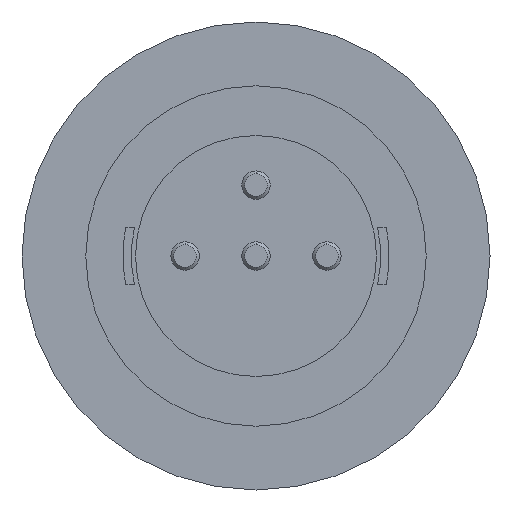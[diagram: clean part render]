
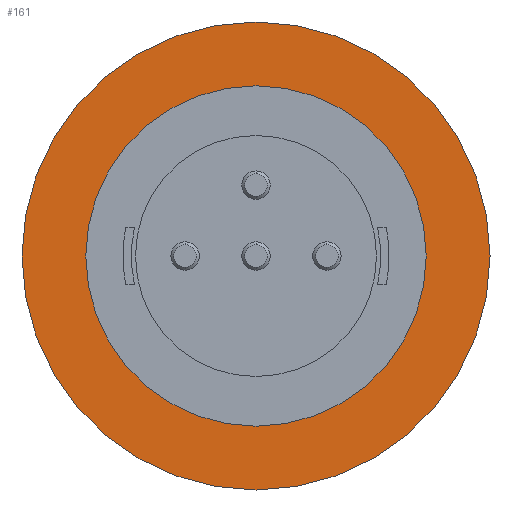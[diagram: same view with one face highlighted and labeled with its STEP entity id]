
A CAD part, front view. The second image highlights one B-rep face of the part: STEP entity #161.
In plain terms, the highlighted planar face has unit normal (0, -1, 0).
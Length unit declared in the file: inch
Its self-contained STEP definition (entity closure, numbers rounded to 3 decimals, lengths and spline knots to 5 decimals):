
#27 = ORIENTED_EDGE ( 'NONE', *, *, #752, .T. ) ;
#47 = AXIS2_PLACEMENT_3D ( 'NONE', #1743, #1665, #1512 ) ;
#58 = CARTESIAN_POINT ( 'NONE',  ( 0., -3.1, 0. ) ) ;
#77 = DIRECTION ( 'NONE',  ( 0., -1., 0. ) ) ;
#83 = AXIS2_PLACEMENT_3D ( 'NONE', #1398, #424, #1243 ) ;
#161 = ADVANCED_FACE ( 'NONE', ( #200, #1588 ), #606, .T. ) ;
#200 = FACE_BOUND ( 'NONE', #368, .T. ) ;
#220 = CARTESIAN_POINT ( 'NONE',  ( 0., -3.1, 8.25 ) ) ;
#285 = CIRCLE ( 'NONE', #1160, 8.25 ) ;
#323 = ORIENTED_EDGE ( 'NONE', *, *, #815, .F. ) ;
#343 = CARTESIAN_POINT ( 'NONE',  ( 0., -3.1, 0. ) ) ;
#368 = EDGE_LOOP ( 'NONE', ( #323, #373 ) ) ;
#373 = ORIENTED_EDGE ( 'NONE', *, *, #448, .F. ) ;
#424 = DIRECTION ( 'NONE',  ( 0., -1., 0. ) ) ;
#448 = EDGE_CURVE ( 'NONE', #1286, #1372, #1666, .T. ) ;
#471 = CARTESIAN_POINT ( 'NONE',  ( 0., -3.1, -8.25 ) ) ;
#606 = PLANE ( 'NONE',  #1515 ) ;
#752 = EDGE_CURVE ( 'NONE', #952, #1498, #285, .T. ) ;
#815 = EDGE_CURVE ( 'NONE', #1372, #1286, #1256, .T. ) ;
#898 = DIRECTION ( 'NONE',  ( 0., 0., -1. ) ) ;
#952 = VERTEX_POINT ( 'NONE', #471 ) ;
#963 = CARTESIAN_POINT ( 'NONE',  ( 0., -3.1, -6. ) ) ;
#1055 = EDGE_LOOP ( 'NONE', ( #1130, #27 ) ) ;
#1130 = ORIENTED_EDGE ( 'NONE', *, *, #1779, .T. ) ;
#1156 = CARTESIAN_POINT ( 'NONE',  ( 0., -3.1, 0. ) ) ;
#1160 = AXIS2_PLACEMENT_3D ( 'NONE', #343, #77, #1209 ) ;
#1193 = DIRECTION ( 'NONE',  ( 0., -1., 0. ) ) ;
#1209 = DIRECTION ( 'NONE',  ( 0., 0., -1. ) ) ;
#1243 = DIRECTION ( 'NONE',  ( 0., 0., -1. ) ) ;
#1256 = CIRCLE ( 'NONE', #47, 6. ) ;
#1283 = AXIS2_PLACEMENT_3D ( 'NONE', #1156, #1193, #1751 ) ;
#1286 = VERTEX_POINT ( 'NONE', #963 ) ;
#1307 = DIRECTION ( 'NONE',  ( 0., -1., 0. ) ) ;
#1372 = VERTEX_POINT ( 'NONE', #1787 ) ;
#1398 = CARTESIAN_POINT ( 'NONE',  ( 0., -3.1, 0. ) ) ;
#1498 = VERTEX_POINT ( 'NONE', #220 ) ;
#1512 = DIRECTION ( 'NONE',  ( 0., 0., -1. ) ) ;
#1515 = AXIS2_PLACEMENT_3D ( 'NONE', #58, #1307, #898 ) ;
#1588 = FACE_OUTER_BOUND ( 'NONE', #1055, .T. ) ;
#1596 = CIRCLE ( 'NONE', #1283, 8.25 ) ;
#1665 = DIRECTION ( 'NONE',  ( 0., -1., 0. ) ) ;
#1666 = CIRCLE ( 'NONE', #83, 6. ) ;
#1743 = CARTESIAN_POINT ( 'NONE',  ( 0., -3.1, 0. ) ) ;
#1751 = DIRECTION ( 'NONE',  ( 0., 0., -1. ) ) ;
#1779 = EDGE_CURVE ( 'NONE', #1498, #952, #1596, .T. ) ;
#1787 = CARTESIAN_POINT ( 'NONE',  ( 0., -3.1, 6. ) ) ;
